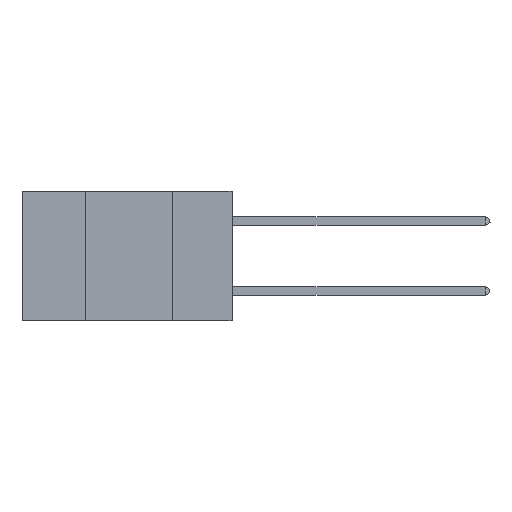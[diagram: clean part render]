
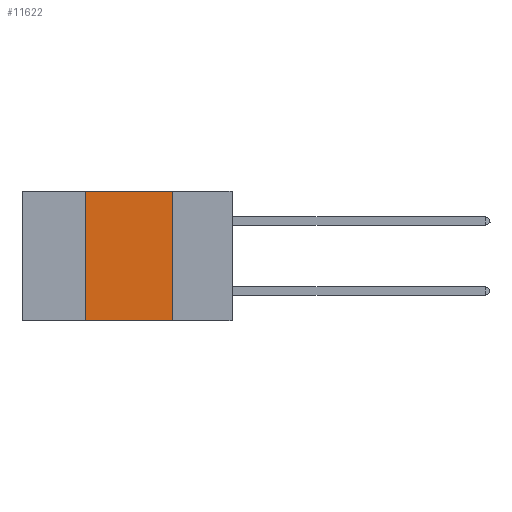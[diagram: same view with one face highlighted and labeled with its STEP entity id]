
A CAD part, left-side view. The second image highlights one B-rep face of the part: STEP entity #11622.
In plain terms, the highlighted planar face has unit normal (-1, 0, 0).
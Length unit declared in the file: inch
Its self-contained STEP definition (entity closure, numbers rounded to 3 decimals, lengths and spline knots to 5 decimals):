
#80 = ORIENTED_EDGE ( 'NONE', *, *, #3996, .T. ) ;
#724 = EDGE_CURVE ( 'NONE', #10964, #13774, #5988, .T. ) ;
#1284 = LINE ( 'NONE', #13471, #18345 ) ;
#1345 = PLANE ( 'NONE',  #8332 ) ;
#3985 = EDGE_CURVE ( 'NONE', #13774, #18452, #11428, .T. ) ;
#3996 = EDGE_CURVE ( 'NONE', #10964, #7290, #15742, .T. ) ;
#4672 = DIRECTION ( 'NONE',  ( 1., 0., 0. ) ) ;
#5163 = DIRECTION ( 'NONE',  ( 0., -1., 0. ) ) ;
#5614 = ORIENTED_EDGE ( 'NONE', *, *, #16836, .F. ) ;
#5988 = LINE ( 'NONE', #16862, #12141 ) ;
#7178 = VECTOR ( 'NONE', #5163, 39.37008 ) ;
#7242 = ORIENTED_EDGE ( 'NONE', *, *, #724, .F. ) ;
#7290 = VERTEX_POINT ( 'NONE', #14375 ) ;
#7483 = DIRECTION ( 'NONE',  ( 0., 0., -1. ) ) ;
#8093 = CARTESIAN_POINT ( 'NONE',  ( 0., 0.6, -0.37 ) ) ;
#8193 = DIRECTION ( 'NONE',  ( 0., -1., 0. ) ) ;
#8332 = AXIS2_PLACEMENT_3D ( 'NONE', #15453, #4672, #7483 ) ;
#8989 = CARTESIAN_POINT ( 'NONE',  ( 0., 0.17, 0. ) ) ;
#9173 = ORIENTED_EDGE ( 'NONE', *, *, #3985, .F. ) ;
#10431 = DIRECTION ( 'NONE',  ( 0., 0., 1. ) ) ;
#10964 = VERTEX_POINT ( 'NONE', #16482 ) ;
#11428 = LINE ( 'NONE', #12914, #17809 ) ;
#11622 = ADVANCED_FACE ( 'NONE', ( #15149 ), #1345, .F. ) ;
#12141 = VECTOR ( 'NONE', #10431, 39.37008 ) ;
#12914 = CARTESIAN_POINT ( 'NONE',  ( 0., 0.6, 0. ) ) ;
#13471 = CARTESIAN_POINT ( 'NONE',  ( 0., 0.17, 0. ) ) ;
#13774 = VERTEX_POINT ( 'NONE', #16609 ) ;
#14375 = CARTESIAN_POINT ( 'NONE',  ( 0., 0.17, -0.37 ) ) ;
#15149 = FACE_OUTER_BOUND ( 'NONE', #15439, .T. ) ;
#15439 = EDGE_LOOP ( 'NONE', ( #5614, #9173, #7242, #80 ) ) ;
#15453 = CARTESIAN_POINT ( 'NONE',  ( 0., 0.6, 0. ) ) ;
#15742 = LINE ( 'NONE', #8093, #7178 ) ;
#16482 = CARTESIAN_POINT ( 'NONE',  ( 0., 0.42, -0.37 ) ) ;
#16609 = CARTESIAN_POINT ( 'NONE',  ( 0., 0.42, 0. ) ) ;
#16836 = EDGE_CURVE ( 'NONE', #18452, #7290, #1284, .T. ) ;
#16862 = CARTESIAN_POINT ( 'NONE',  ( 0., 0.42, 0. ) ) ;
#17809 = VECTOR ( 'NONE', #8193, 39.37008 ) ;
#18345 = VECTOR ( 'NONE', #19700, 39.37008 ) ;
#18452 = VERTEX_POINT ( 'NONE', #8989 ) ;
#19700 = DIRECTION ( 'NONE',  ( 0., 0., -1. ) ) ;
